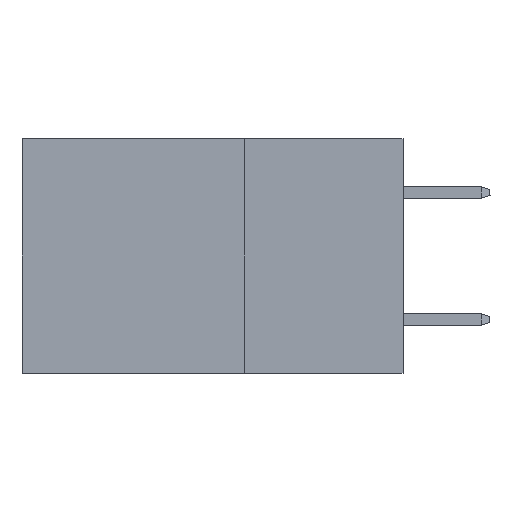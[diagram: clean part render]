
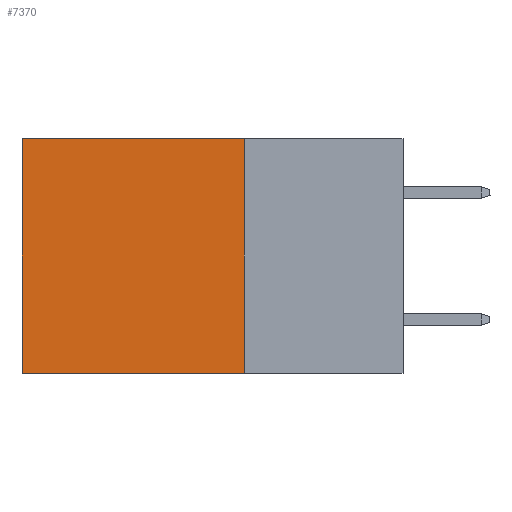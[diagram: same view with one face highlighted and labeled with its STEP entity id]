
A CAD part, left-side view. The second image highlights one B-rep face of the part: STEP entity #7370.
In plain terms, the highlighted planar face has unit normal (-1, 0, 0).
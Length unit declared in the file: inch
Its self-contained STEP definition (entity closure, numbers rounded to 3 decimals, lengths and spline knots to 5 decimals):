
#2438 = DIRECTION ( 'NONE',  ( 0., 0., -1. ) ) ;
#2448 = EDGE_CURVE ( 'NONE', #3681, #6496, #36491, .T. ) ;
#3341 = EDGE_LOOP ( 'NONE', ( #4378, #33861, #15440, #20898 ) ) ;
#3681 = VERTEX_POINT ( 'NONE', #8037 ) ;
#4378 = ORIENTED_EDGE ( 'NONE', *, *, #18445, .T. ) ;
#4608 = LINE ( 'NONE', #27439, #36324 ) ;
#5124 = CARTESIAN_POINT ( 'NONE',  ( 0.2875, 0.6, 0. ) ) ;
#6496 = VERTEX_POINT ( 'NONE', #17392 ) ;
#7370 = ADVANCED_FACE ( 'NONE', ( #7572 ), #10381, .F. ) ;
#7572 = FACE_OUTER_BOUND ( 'NONE', #3341, .T. ) ;
#7793 = CARTESIAN_POINT ( 'NONE',  ( 0.2875, 0.25, 0. ) ) ;
#8037 = CARTESIAN_POINT ( 'NONE',  ( 0.2875, 0.25, 0. ) ) ;
#10381 = PLANE ( 'NONE',  #27216 ) ;
#11701 = LINE ( 'NONE', #12250, #15334 ) ;
#12250 = CARTESIAN_POINT ( 'NONE',  ( 0.2875, 0.25, -0.37 ) ) ;
#14883 = VECTOR ( 'NONE', #33057, 39.37008 ) ;
#15334 = VECTOR ( 'NONE', #23122, 39.37008 ) ;
#15440 = ORIENTED_EDGE ( 'NONE', *, *, #2448, .F. ) ;
#15684 = EDGE_CURVE ( 'NONE', #6496, #20258, #11701, .T. ) ;
#17392 = CARTESIAN_POINT ( 'NONE',  ( 0.2875, 0.25, -0.37 ) ) ;
#18445 = EDGE_CURVE ( 'NONE', #20292, #20258, #4608, .T. ) ;
#19021 = LINE ( 'NONE', #7793, #14883 ) ;
#19382 = DIRECTION ( 'NONE',  ( 0., 0., -1. ) ) ;
#20258 = VERTEX_POINT ( 'NONE', #35878 ) ;
#20292 = VERTEX_POINT ( 'NONE', #5124 ) ;
#20898 = ORIENTED_EDGE ( 'NONE', *, *, #28439, .T. ) ;
#22540 = DIRECTION ( 'NONE',  ( 1., 0., 0. ) ) ;
#23122 = DIRECTION ( 'NONE',  ( 0., 1., 0. ) ) ;
#25345 = CARTESIAN_POINT ( 'NONE',  ( 0.2875, 0.25, 0. ) ) ;
#27216 = AXIS2_PLACEMENT_3D ( 'NONE', #25345, #22540, #27775 ) ;
#27439 = CARTESIAN_POINT ( 'NONE',  ( 0.2875, 0.6, 0. ) ) ;
#27775 = DIRECTION ( 'NONE',  ( 0., 0., -1. ) ) ;
#28439 = EDGE_CURVE ( 'NONE', #3681, #20292, #19021, .T. ) ;
#29169 = VECTOR ( 'NONE', #2438, 39.37008 ) ;
#33057 = DIRECTION ( 'NONE',  ( 0., 1., 0. ) ) ;
#33303 = CARTESIAN_POINT ( 'NONE',  ( 0.2875, 0.25, 0. ) ) ;
#33861 = ORIENTED_EDGE ( 'NONE', *, *, #15684, .F. ) ;
#35878 = CARTESIAN_POINT ( 'NONE',  ( 0.2875, 0.6, -0.37 ) ) ;
#36324 = VECTOR ( 'NONE', #19382, 39.37008 ) ;
#36491 = LINE ( 'NONE', #33303, #29169 ) ;
